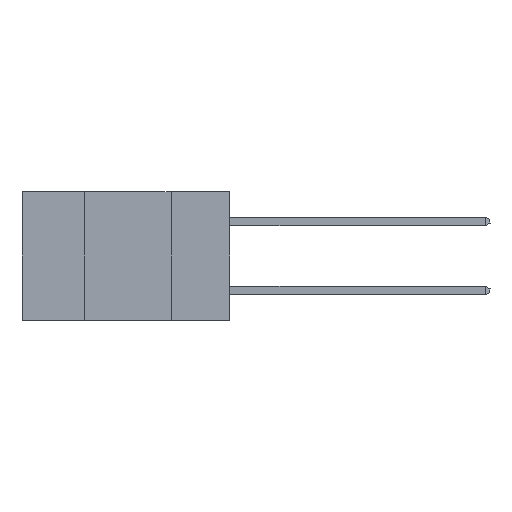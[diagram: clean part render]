
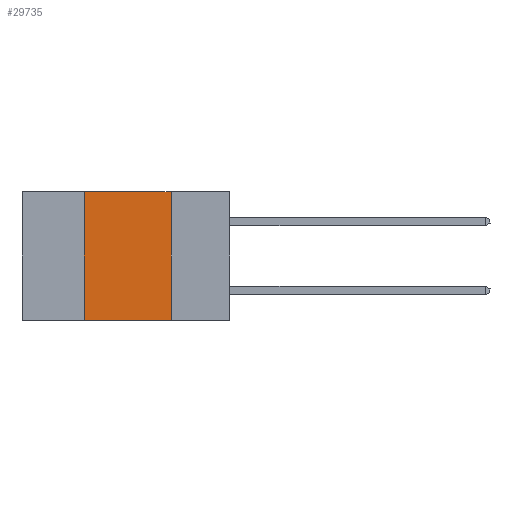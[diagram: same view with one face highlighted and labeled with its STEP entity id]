
A CAD part, left-side view. The second image highlights one B-rep face of the part: STEP entity #29735.
In plain terms, the highlighted planar face has unit normal (-1, 0, 0).
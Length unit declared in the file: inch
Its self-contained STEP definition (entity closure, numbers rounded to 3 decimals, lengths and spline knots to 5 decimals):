
#2622 = VECTOR ( 'NONE', #27945, 39.37008 ) ;
#2678 = LINE ( 'NONE', #8272, #20016 ) ;
#3587 = VECTOR ( 'NONE', #6376, 39.37008 ) ;
#3655 = CARTESIAN_POINT ( 'NONE',  ( 0., 0.6, 0. ) ) ;
#4362 = ORIENTED_EDGE ( 'NONE', *, *, #20964, .F. ) ;
#4994 = VERTEX_POINT ( 'NONE', #7679 ) ;
#5085 = CARTESIAN_POINT ( 'NONE',  ( 0., 0.6, -0.37 ) ) ;
#5468 = AXIS2_PLACEMENT_3D ( 'NONE', #8780, #24988, #29800 ) ;
#6376 = DIRECTION ( 'NONE',  ( 0., -1., 0. ) ) ;
#6895 = VECTOR ( 'NONE', #10868, 39.37008 ) ;
#7679 = CARTESIAN_POINT ( 'NONE',  ( 0., 0.42, -0.37 ) ) ;
#7695 = LINE ( 'NONE', #5085, #2622 ) ;
#8272 = CARTESIAN_POINT ( 'NONE',  ( 0., 0.17, 0. ) ) ;
#8691 = VERTEX_POINT ( 'NONE', #27353 ) ;
#8709 = EDGE_CURVE ( 'NONE', #4994, #8691, #19480, .T. ) ;
#8780 = CARTESIAN_POINT ( 'NONE',  ( 0., 0.6, 0. ) ) ;
#8987 = PLANE ( 'NONE',  #5468 ) ;
#9371 = CARTESIAN_POINT ( 'NONE',  ( 0., 0.17, -0.37 ) ) ;
#10566 = DIRECTION ( 'NONE',  ( 0., 0., -1. ) ) ;
#10868 = DIRECTION ( 'NONE',  ( 0., 0., 1. ) ) ;
#12265 = ORIENTED_EDGE ( 'NONE', *, *, #8709, .F. ) ;
#12275 = EDGE_CURVE ( 'NONE', #27116, #19288, #2678, .T. ) ;
#14591 = CARTESIAN_POINT ( 'NONE',  ( 0., 0.17, 0. ) ) ;
#14906 = ORIENTED_EDGE ( 'NONE', *, *, #25276, .T. ) ;
#18449 = FACE_OUTER_BOUND ( 'NONE', #21664, .T. ) ;
#19288 = VERTEX_POINT ( 'NONE', #9371 ) ;
#19480 = LINE ( 'NONE', #24969, #6895 ) ;
#20016 = VECTOR ( 'NONE', #10566, 39.37008 ) ;
#20964 = EDGE_CURVE ( 'NONE', #8691, #27116, #28912, .T. ) ;
#21664 = EDGE_LOOP ( 'NONE', ( #27991, #4362, #12265, #14906 ) ) ;
#24969 = CARTESIAN_POINT ( 'NONE',  ( 0., 0.42, 0. ) ) ;
#24988 = DIRECTION ( 'NONE',  ( 1., 0., 0. ) ) ;
#25276 = EDGE_CURVE ( 'NONE', #4994, #19288, #7695, .T. ) ;
#27116 = VERTEX_POINT ( 'NONE', #14591 ) ;
#27353 = CARTESIAN_POINT ( 'NONE',  ( 0., 0.42, 0. ) ) ;
#27945 = DIRECTION ( 'NONE',  ( 0., -1., 0. ) ) ;
#27991 = ORIENTED_EDGE ( 'NONE', *, *, #12275, .F. ) ;
#28912 = LINE ( 'NONE', #3655, #3587 ) ;
#29735 = ADVANCED_FACE ( 'NONE', ( #18449 ), #8987, .F. ) ;
#29800 = DIRECTION ( 'NONE',  ( 0., 0., -1. ) ) ;
